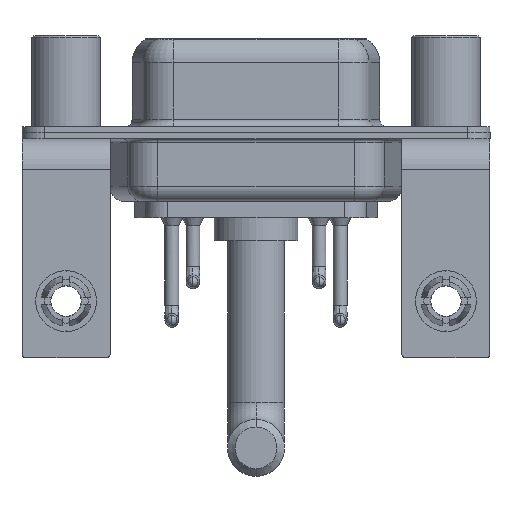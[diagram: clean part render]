
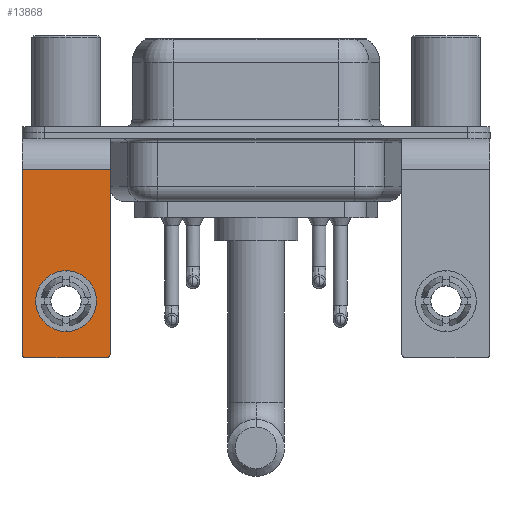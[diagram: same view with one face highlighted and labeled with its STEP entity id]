
A CAD part, front view. The second image highlights one B-rep face of the part: STEP entity #13868.
In plain terms, the highlighted planar face has unit normal (0, -1, 0).
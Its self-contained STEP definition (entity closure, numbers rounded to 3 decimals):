
#290 = AXIS2_PLACEMENT_3D ( 'NONE', #12279, #18900, #4750 ) ;
#602 = CARTESIAN_POINT ( 'NONE',  ( 0., -6.25, -9.07 ) ) ;
#729 = AXIS2_PLACEMENT_3D ( 'NONE', #13710, #991, #13605 ) ;
#991 = DIRECTION ( 'NONE',  ( 0., -1., 0. ) ) ;
#1142 = FACE_OUTER_BOUND ( 'NONE', #14519, .T. ) ;
#1479 = CARTESIAN_POINT ( 'NONE',  ( 2.9, -6.25, -14.8 ) ) ;
#2000 = EDGE_CURVE ( 'NONE', #19638, #5973, #12676, .T. ) ;
#2110 = VERTEX_POINT ( 'NONE', #2229 ) ;
#2229 = CARTESIAN_POINT ( 'NONE',  ( 2.9, -6.25, -2.4 ) ) ;
#2262 = CIRCLE ( 'NONE', #290, 2. ) ;
#2375 = CIRCLE ( 'NONE', #18560, 2. ) ;
#2533 = VERTEX_POINT ( 'NONE', #19076 ) ;
#2625 = VECTOR ( 'NONE', #10955, 1000. ) ;
#2696 = CARTESIAN_POINT ( 'NONE',  ( 2.9, -6.25, -2.4 ) ) ;
#2707 = EDGE_CURVE ( 'NONE', #18337, #10450, #7753, .T. ) ;
#2899 = VERTEX_POINT ( 'NONE', #602 ) ;
#3250 = DIRECTION ( 'NONE',  ( 0., 1., 0. ) ) ;
#3433 = VECTOR ( 'NONE', #11109, 1000. ) ;
#3489 = DIRECTION ( 'NONE',  ( 0., 0., 1. ) ) ;
#3627 = ORIENTED_EDGE ( 'NONE', *, *, #4363, .F. ) ;
#4363 = EDGE_CURVE ( 'NONE', #19638, #14549, #10899, .T. ) ;
#4469 = PLANE ( 'NONE',  #6116 ) ;
#4750 = DIRECTION ( 'NONE',  ( 0., 0., 1. ) ) ;
#5875 = DIRECTION ( 'NONE',  ( -1., 0., 0. ) ) ;
#5973 = VERTEX_POINT ( 'NONE', #13928 ) ;
#6019 = EDGE_CURVE ( 'NONE', #2899, #2533, #2262, .T. ) ;
#6116 = AXIS2_PLACEMENT_3D ( 'NONE', #2696, #9108, #13965 ) ;
#6421 = AXIS2_PLACEMENT_3D ( 'NONE', #6494, #19200, #3489 ) ;
#6494 = CARTESIAN_POINT ( 'NONE',  ( 2.65, -6.25, -14.55 ) ) ;
#6604 = CARTESIAN_POINT ( 'NONE',  ( -2.9, -6.25, -2.4 ) ) ;
#7120 = CARTESIAN_POINT ( 'NONE',  ( 2.9, -6.25, -2.4 ) ) ;
#7228 = CARTESIAN_POINT ( 'NONE',  ( 2.65, -6.25, -14.8 ) ) ;
#7613 = LINE ( 'NONE', #13704, #9981 ) ;
#7653 = EDGE_CURVE ( 'NONE', #2110, #5973, #18270, .T. ) ;
#7753 = LINE ( 'NONE', #9397, #2625 ) ;
#8006 = CARTESIAN_POINT ( 'NONE',  ( 0., -6.25, -11.07 ) ) ;
#8484 = ORIENTED_EDGE ( 'NONE', *, *, #2707, .T. ) ;
#8894 = ORIENTED_EDGE ( 'NONE', *, *, #9929, .T. ) ;
#9020 = ORIENTED_EDGE ( 'NONE', *, *, #9800, .T. ) ;
#9108 = DIRECTION ( 'NONE',  ( 0., 1., 0. ) ) ;
#9397 = CARTESIAN_POINT ( 'NONE',  ( -2.9, -6.25, -2.4 ) ) ;
#9800 = EDGE_CURVE ( 'NONE', #10450, #14549, #11317, .T. ) ;
#9929 = EDGE_CURVE ( 'NONE', #2533, #2899, #2375, .T. ) ;
#9981 = VECTOR ( 'NONE', #5875, 1000. ) ;
#10450 = VERTEX_POINT ( 'NONE', #12991 ) ;
#10861 = ORIENTED_EDGE ( 'NONE', *, *, #2000, .T. ) ;
#10899 = LINE ( 'NONE', #1479, #3433 ) ;
#10955 = DIRECTION ( 'NONE',  ( 0., 0., -1. ) ) ;
#10976 = CARTESIAN_POINT ( 'NONE',  ( -2.65, -6.25, -14.8 ) ) ;
#11109 = DIRECTION ( 'NONE',  ( -1., 0., 0. ) ) ;
#11317 = CIRCLE ( 'NONE', #729, 0.25 ) ;
#11716 = EDGE_CURVE ( 'NONE', #2110, #18337, #7613, .T. ) ;
#12228 = VECTOR ( 'NONE', #19723, 1000. ) ;
#12279 = CARTESIAN_POINT ( 'NONE',  ( 0., -6.25, -11.07 ) ) ;
#12676 = CIRCLE ( 'NONE', #6421, 0.25 ) ;
#12950 = DIRECTION ( 'NONE',  ( 0., 0., 1. ) ) ;
#12991 = CARTESIAN_POINT ( 'NONE',  ( -2.9, -6.25, -14.55 ) ) ;
#13236 = ORIENTED_EDGE ( 'NONE', *, *, #7653, .F. ) ;
#13605 = DIRECTION ( 'NONE',  ( 0., 0., 1. ) ) ;
#13704 = CARTESIAN_POINT ( 'NONE',  ( 2.9, -6.25, -2.4 ) ) ;
#13710 = CARTESIAN_POINT ( 'NONE',  ( -2.65, -6.25, -14.55 ) ) ;
#13868 = ADVANCED_FACE ( 'NONE', ( #16874, #1142 ), #4469, .F. ) ;
#13928 = CARTESIAN_POINT ( 'NONE',  ( 2.9, -6.25, -14.55 ) ) ;
#13965 = DIRECTION ( 'NONE',  ( 0., 0., 1. ) ) ;
#14519 = EDGE_LOOP ( 'NONE', ( #8484, #9020, #3627, #10861, #13236, #18563 ) ) ;
#14549 = VERTEX_POINT ( 'NONE', #10976 ) ;
#15232 = ORIENTED_EDGE ( 'NONE', *, *, #6019, .T. ) ;
#15584 = EDGE_LOOP ( 'NONE', ( #8894, #15232 ) ) ;
#16874 = FACE_BOUND ( 'NONE', #15584, .T. ) ;
#18270 = LINE ( 'NONE', #7120, #12228 ) ;
#18337 = VERTEX_POINT ( 'NONE', #6604 ) ;
#18560 = AXIS2_PLACEMENT_3D ( 'NONE', #8006, #3250, #12950 ) ;
#18563 = ORIENTED_EDGE ( 'NONE', *, *, #11716, .T. ) ;
#18900 = DIRECTION ( 'NONE',  ( 0., 1., 0. ) ) ;
#19076 = CARTESIAN_POINT ( 'NONE',  ( 0., -6.25, -13.07 ) ) ;
#19200 = DIRECTION ( 'NONE',  ( 0., -1., 0. ) ) ;
#19638 = VERTEX_POINT ( 'NONE', #7228 ) ;
#19723 = DIRECTION ( 'NONE',  ( 0., 0., -1. ) ) ;
